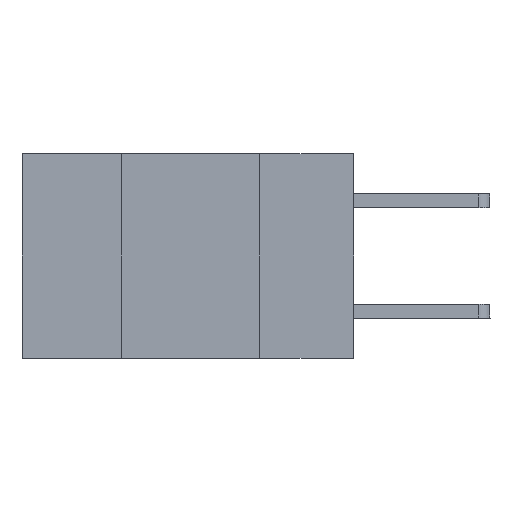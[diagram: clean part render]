
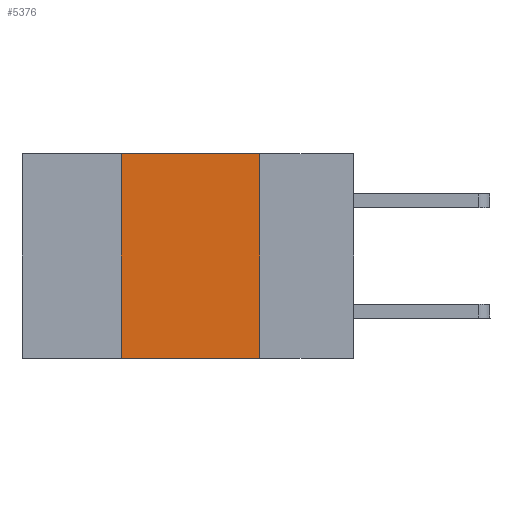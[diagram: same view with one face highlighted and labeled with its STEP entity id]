
A CAD part, left-side view. The second image highlights one B-rep face of the part: STEP entity #5376.
In plain terms, the highlighted planar face has unit normal (-1, 0, 0).
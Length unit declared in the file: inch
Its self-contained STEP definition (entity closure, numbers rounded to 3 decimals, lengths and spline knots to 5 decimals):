
#432 = VERTEX_POINT ( 'NONE', #7535 ) ;
#727 = DIRECTION ( 'NONE',  ( 0., 0., -1. ) ) ;
#1899 = DIRECTION ( 'NONE',  ( 0., -1., 0. ) ) ;
#1958 = CARTESIAN_POINT ( 'NONE',  ( 0., 0.42, 0. ) ) ;
#2101 = VERTEX_POINT ( 'NONE', #4305 ) ;
#2144 = AXIS2_PLACEMENT_3D ( 'NONE', #3796, #6734, #727 ) ;
#2162 = EDGE_CURVE ( 'NONE', #2101, #432, #3513, .T. ) ;
#2397 = EDGE_CURVE ( 'NONE', #11013, #432, #6271, .T. ) ;
#3513 = LINE ( 'NONE', #10207, #8138 ) ;
#3787 = VERTEX_POINT ( 'NONE', #1958 ) ;
#3796 = CARTESIAN_POINT ( 'NONE',  ( 0., 0.6, 0. ) ) ;
#4305 = CARTESIAN_POINT ( 'NONE',  ( 0., 0.17, 0. ) ) ;
#4393 = VECTOR ( 'NONE', #11898, 39.37008 ) ;
#4598 = ORIENTED_EDGE ( 'NONE', *, *, #6399, .F. ) ;
#4707 = LINE ( 'NONE', #10963, #4393 ) ;
#5014 = EDGE_LOOP ( 'NONE', ( #6867, #12026, #4598, #10081 ) ) ;
#5191 = CARTESIAN_POINT ( 'NONE',  ( 0., 0.42, -0.37 ) ) ;
#5319 = DIRECTION ( 'NONE',  ( 0., 0., 1. ) ) ;
#5376 = ADVANCED_FACE ( 'NONE', ( #11311 ), #12528, .F. ) ;
#6271 = LINE ( 'NONE', #8813, #8276 ) ;
#6399 = EDGE_CURVE ( 'NONE', #11013, #3787, #11718, .T. ) ;
#6523 = VECTOR ( 'NONE', #5319, 39.37008 ) ;
#6734 = DIRECTION ( 'NONE',  ( 1., 0., 0. ) ) ;
#6867 = ORIENTED_EDGE ( 'NONE', *, *, #2162, .F. ) ;
#7535 = CARTESIAN_POINT ( 'NONE',  ( 0., 0.17, -0.37 ) ) ;
#8138 = VECTOR ( 'NONE', #11264, 39.37008 ) ;
#8276 = VECTOR ( 'NONE', #1899, 39.37008 ) ;
#8813 = CARTESIAN_POINT ( 'NONE',  ( 0., 0.6, -0.37 ) ) ;
#10081 = ORIENTED_EDGE ( 'NONE', *, *, #2397, .T. ) ;
#10207 = CARTESIAN_POINT ( 'NONE',  ( 0., 0.17, 0. ) ) ;
#10963 = CARTESIAN_POINT ( 'NONE',  ( 0., 0.6, 0. ) ) ;
#11013 = VERTEX_POINT ( 'NONE', #5191 ) ;
#11264 = DIRECTION ( 'NONE',  ( 0., 0., -1. ) ) ;
#11311 = FACE_OUTER_BOUND ( 'NONE', #5014, .T. ) ;
#11514 = EDGE_CURVE ( 'NONE', #3787, #2101, #4707, .T. ) ;
#11718 = LINE ( 'NONE', #12049, #6523 ) ;
#11898 = DIRECTION ( 'NONE',  ( 0., -1., 0. ) ) ;
#12026 = ORIENTED_EDGE ( 'NONE', *, *, #11514, .F. ) ;
#12049 = CARTESIAN_POINT ( 'NONE',  ( 0., 0.42, 0. ) ) ;
#12528 = PLANE ( 'NONE',  #2144 ) ;
